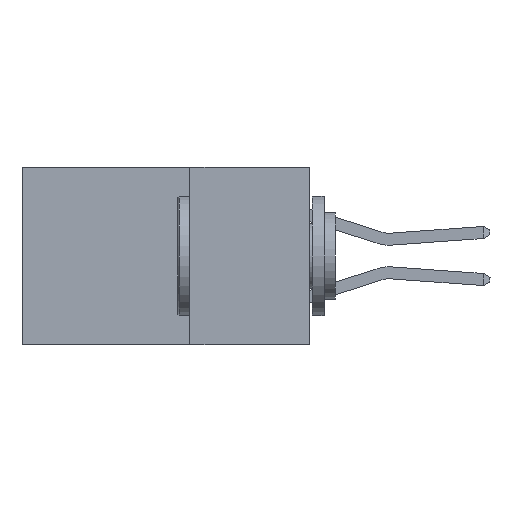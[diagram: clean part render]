
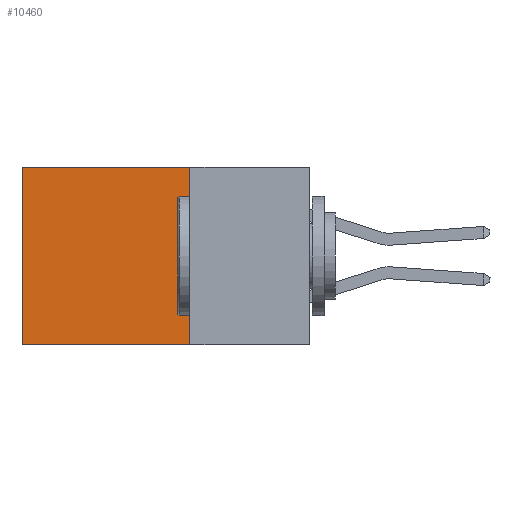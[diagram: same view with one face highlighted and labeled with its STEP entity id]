
A CAD part, left-side view. The second image highlights one B-rep face of the part: STEP entity #10460.
In plain terms, the highlighted planar face has unit normal (-1, 0, 0).
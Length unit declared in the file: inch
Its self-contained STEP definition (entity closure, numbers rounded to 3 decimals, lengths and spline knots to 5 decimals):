
#629 = LINE ( 'NONE', #19464, #10932 ) ;
#876 = CARTESIAN_POINT ( 'NONE',  ( 0.298, 0.25, 0. ) ) ;
#1960 = ORIENTED_EDGE ( 'NONE', *, *, #10626, .T. ) ;
#2190 = CARTESIAN_POINT ( 'NONE',  ( 0.298, 0.25, 0. ) ) ;
#2384 = PLANE ( 'NONE',  #7888 ) ;
#3052 = EDGE_CURVE ( 'NONE', #5577, #7794, #16200, .T. ) ;
#3874 = DIRECTION ( 'NONE',  ( 0., 0., -1. ) ) ;
#4043 = DIRECTION ( 'NONE',  ( 0., 0., -1. ) ) ;
#4342 = CARTESIAN_POINT ( 'NONE',  ( 0.298, 0.25, 0. ) ) ;
#4586 = LINE ( 'NONE', #15789, #8186 ) ;
#4628 = CARTESIAN_POINT ( 'NONE',  ( 0.298, 0.25, -0.37 ) ) ;
#5577 = VERTEX_POINT ( 'NONE', #4342 ) ;
#6071 = CARTESIAN_POINT ( 'NONE',  ( 0.298, 0.25, -0.37 ) ) ;
#6759 = ORIENTED_EDGE ( 'NONE', *, *, #17673, .F. ) ;
#7794 = VERTEX_POINT ( 'NONE', #4628 ) ;
#7888 = AXIS2_PLACEMENT_3D ( 'NONE', #2190, #14317, #3874 ) ;
#8186 = VECTOR ( 'NONE', #9879, 39.37008 ) ;
#9381 = LINE ( 'NONE', #6071, #14572 ) ;
#9879 = DIRECTION ( 'NONE',  ( 0., 1., 0. ) ) ;
#10035 = VERTEX_POINT ( 'NONE', #19212 ) ;
#10460 = ADVANCED_FACE ( 'NONE', ( #12163 ), #2384, .F. ) ;
#10626 = EDGE_CURVE ( 'NONE', #10035, #12434, #629, .T. ) ;
#10782 = CARTESIAN_POINT ( 'NONE',  ( 0.298, 0.6, -0.37 ) ) ;
#10932 = VECTOR ( 'NONE', #16178, 39.37008 ) ;
#11151 = EDGE_LOOP ( 'NONE', ( #1960, #6759, #19073, #15722 ) ) ;
#12163 = FACE_OUTER_BOUND ( 'NONE', #11151, .T. ) ;
#12434 = VERTEX_POINT ( 'NONE', #10782 ) ;
#13893 = EDGE_CURVE ( 'NONE', #5577, #10035, #4586, .T. ) ;
#14317 = DIRECTION ( 'NONE',  ( 1., 0., 0. ) ) ;
#14572 = VECTOR ( 'NONE', #18112, 39.37008 ) ;
#15722 = ORIENTED_EDGE ( 'NONE', *, *, #13893, .T. ) ;
#15732 = VECTOR ( 'NONE', #4043, 39.37008 ) ;
#15789 = CARTESIAN_POINT ( 'NONE',  ( 0.298, 0.25, 0. ) ) ;
#16178 = DIRECTION ( 'NONE',  ( 0., 0., -1. ) ) ;
#16200 = LINE ( 'NONE', #876, #15732 ) ;
#17673 = EDGE_CURVE ( 'NONE', #7794, #12434, #9381, .T. ) ;
#18112 = DIRECTION ( 'NONE',  ( 0., 1., 0. ) ) ;
#19073 = ORIENTED_EDGE ( 'NONE', *, *, #3052, .F. ) ;
#19212 = CARTESIAN_POINT ( 'NONE',  ( 0.298, 0.6, 0. ) ) ;
#19464 = CARTESIAN_POINT ( 'NONE',  ( 0.298, 0.6, 0. ) ) ;
